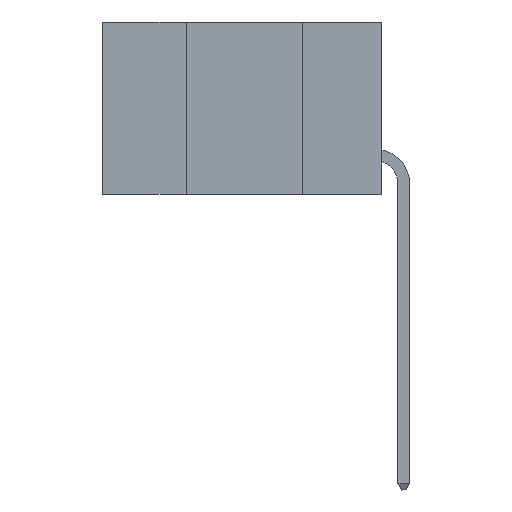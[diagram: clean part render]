
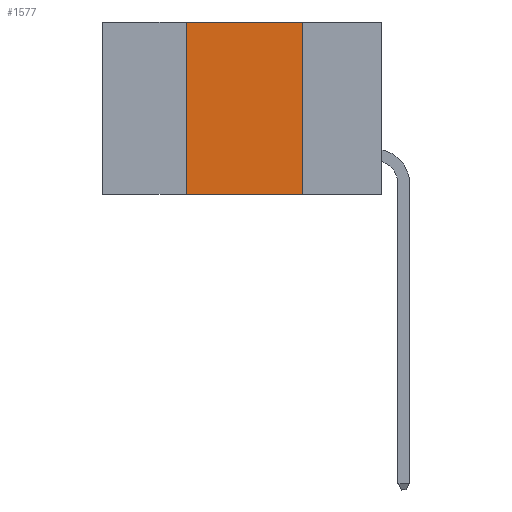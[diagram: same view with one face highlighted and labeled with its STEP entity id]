
A CAD part, left-side view. The second image highlights one B-rep face of the part: STEP entity #1577.
In plain terms, the highlighted planar face has unit normal (-1, 0, 0).
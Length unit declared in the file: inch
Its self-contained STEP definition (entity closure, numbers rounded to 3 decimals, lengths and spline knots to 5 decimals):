
#166 = FACE_OUTER_BOUND ( 'NONE', #9011, .T. ) ;
#186 = DIRECTION ( 'NONE',  ( 0., 0., -1. ) ) ;
#736 = CARTESIAN_POINT ( 'NONE',  ( 0., 0.42, -0.37 ) ) ;
#1290 = DIRECTION ( 'NONE',  ( 0., 0., -1. ) ) ;
#1506 = ORIENTED_EDGE ( 'NONE', *, *, #9453, .F. ) ;
#1577 = ADVANCED_FACE ( 'NONE', ( #166 ), #3665, .F. ) ;
#1609 = VECTOR ( 'NONE', #186, 39.37008 ) ;
#1694 = VERTEX_POINT ( 'NONE', #736 ) ;
#1965 = CARTESIAN_POINT ( 'NONE',  ( 0., 0.17, 0. ) ) ;
#1981 = LINE ( 'NONE', #7648, #7978 ) ;
#2521 = DIRECTION ( 'NONE',  ( 0., 0., 1. ) ) ;
#2670 = CARTESIAN_POINT ( 'NONE',  ( 0., 0.17, -0.37 ) ) ;
#2816 = EDGE_CURVE ( 'NONE', #7144, #6029, #3547, .T. ) ;
#2836 = CARTESIAN_POINT ( 'NONE',  ( 0., 0.42, 0. ) ) ;
#3320 = VECTOR ( 'NONE', #7197, 39.37008 ) ;
#3547 = LINE ( 'NONE', #4072, #3320 ) ;
#3665 = PLANE ( 'NONE',  #8200 ) ;
#3727 = CARTESIAN_POINT ( 'NONE',  ( 0., 0.6, 0. ) ) ;
#3939 = ORIENTED_EDGE ( 'NONE', *, *, #6517, .F. ) ;
#4072 = CARTESIAN_POINT ( 'NONE',  ( 0., 0.6, 0. ) ) ;
#4820 = CARTESIAN_POINT ( 'NONE',  ( 0., 0.17, 0. ) ) ;
#4915 = ORIENTED_EDGE ( 'NONE', *, *, #2816, .F. ) ;
#5799 = LINE ( 'NONE', #7162, #7656 ) ;
#5937 = DIRECTION ( 'NONE',  ( 1., 0., 0. ) ) ;
#5979 = LINE ( 'NONE', #4820, #1609 ) ;
#6029 = VERTEX_POINT ( 'NONE', #1965 ) ;
#6371 = EDGE_CURVE ( 'NONE', #1694, #8901, #1981, .T. ) ;
#6517 = EDGE_CURVE ( 'NONE', #6029, #8901, #5979, .T. ) ;
#7144 = VERTEX_POINT ( 'NONE', #2836 ) ;
#7162 = CARTESIAN_POINT ( 'NONE',  ( 0., 0.42, 0. ) ) ;
#7197 = DIRECTION ( 'NONE',  ( 0., -1., 0. ) ) ;
#7648 = CARTESIAN_POINT ( 'NONE',  ( 0., 0.6, -0.37 ) ) ;
#7656 = VECTOR ( 'NONE', #2521, 39.37008 ) ;
#7978 = VECTOR ( 'NONE', #9176, 39.37008 ) ;
#8200 = AXIS2_PLACEMENT_3D ( 'NONE', #3727, #5937, #1290 ) ;
#8901 = VERTEX_POINT ( 'NONE', #2670 ) ;
#9011 = EDGE_LOOP ( 'NONE', ( #3939, #4915, #1506, #9439 ) ) ;
#9176 = DIRECTION ( 'NONE',  ( 0., -1., 0. ) ) ;
#9439 = ORIENTED_EDGE ( 'NONE', *, *, #6371, .T. ) ;
#9453 = EDGE_CURVE ( 'NONE', #1694, #7144, #5799, .T. ) ;
